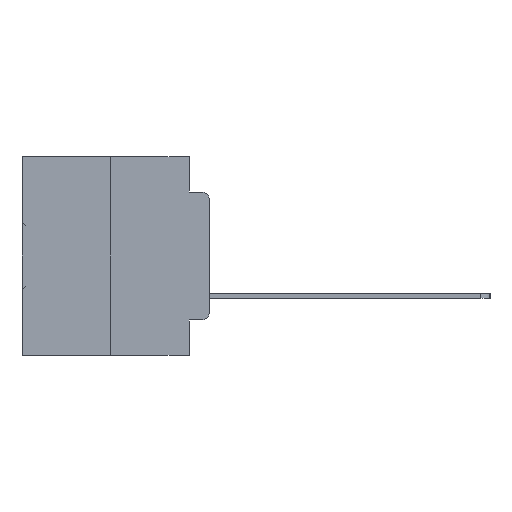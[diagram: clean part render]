
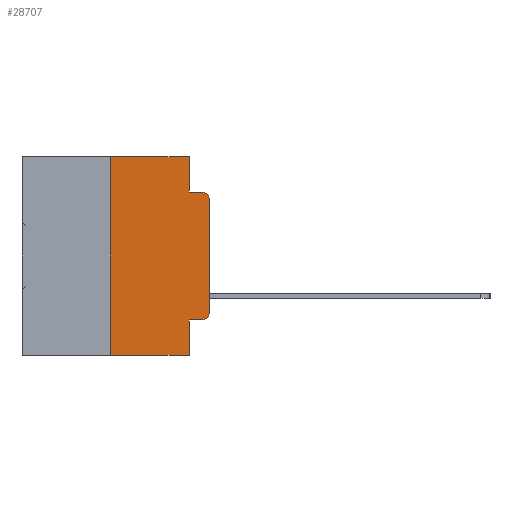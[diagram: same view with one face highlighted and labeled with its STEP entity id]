
A CAD part, left-side view. The second image highlights one B-rep face of the part: STEP entity #28707.
In plain terms, the highlighted planar face has unit normal (-1, 0, 0).
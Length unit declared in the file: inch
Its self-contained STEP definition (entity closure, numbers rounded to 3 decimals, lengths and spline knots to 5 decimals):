
#193 = CARTESIAN_POINT ( 'NONE',  ( 0., 0.051, 0. ) ) ;
#1169 = CIRCLE ( 'NONE', #34010, 0.02 ) ;
#1269 = CARTESIAN_POINT ( 'NONE',  ( 0., 0.473, 0. ) ) ;
#1538 = VECTOR ( 'NONE', #10232, 39.37008 ) ;
#2006 = AXIS2_PLACEMENT_3D ( 'NONE', #13769, #24222, #19014 ) ;
#2078 = CARTESIAN_POINT ( 'NONE',  ( 0., 0.051, -0.0885 ) ) ;
#2983 = DIRECTION ( 'NONE',  ( 0., 0., -1. ) ) ;
#3175 = VECTOR ( 'NONE', #16511, 39.37008 ) ;
#3433 = VECTOR ( 'NONE', #2983, 39.37008 ) ;
#3879 = EDGE_LOOP ( 'NONE', ( #21950, #27041, #23851, #23811, #24262, #24699, #24588, #25602, #26365, #12813 ) ) ;
#4594 = CARTESIAN_POINT ( 'NONE',  ( 0., 0.051, -0.4115 ) ) ;
#4612 = EDGE_CURVE ( 'NONE', #17593, #7597, #31254, .T. ) ;
#4682 = LINE ( 'NONE', #1269, #16323 ) ;
#6451 = EDGE_CURVE ( 'NONE', #7597, #16814, #22571, .T. ) ;
#7597 = VERTEX_POINT ( 'NONE', #2078 ) ;
#8243 = EDGE_CURVE ( 'NONE', #8988, #16814, #1169, .T. ) ;
#8244 = CARTESIAN_POINT ( 'NONE',  ( 0., 0.02, -0.1085 ) ) ;
#8622 = CARTESIAN_POINT ( 'NONE',  ( 0., 0., -0.3915 ) ) ;
#8988 = VERTEX_POINT ( 'NONE', #13660 ) ;
#9167 = CARTESIAN_POINT ( 'NONE',  ( 0., 0.02, -0.3915 ) ) ;
#10001 = LINE ( 'NONE', #22939, #23158 ) ;
#10232 = DIRECTION ( 'NONE',  ( 0., 0., 1. ) ) ;
#10560 = VERTEX_POINT ( 'NONE', #4594 ) ;
#10919 = DIRECTION ( 'NONE',  ( 0., 0., -1. ) ) ;
#11129 = CARTESIAN_POINT ( 'NONE',  ( 0., 0.25, 0. ) ) ;
#11815 = DIRECTION ( 'NONE',  ( 0., 0., -1. ) ) ;
#12265 = LINE ( 'NONE', #193, #3433 ) ;
#12270 = EDGE_CURVE ( 'NONE', #27162, #27237, #26107, .T. ) ;
#12813 = ORIENTED_EDGE ( 'NONE', *, *, #23027, .T. ) ;
#13588 = EDGE_CURVE ( 'NONE', #33265, #8988, #10001, .T. ) ;
#13660 = CARTESIAN_POINT ( 'NONE',  ( 0., 0., -0.1085 ) ) ;
#13769 = CARTESIAN_POINT ( 'NONE',  ( 0., 0.473, 0. ) ) ;
#14404 = CARTESIAN_POINT ( 'NONE',  ( 0., 0.473, -0.5 ) ) ;
#16323 = VECTOR ( 'NONE', #30356, 39.37008 ) ;
#16364 = PLANE ( 'NONE',  #2006 ) ;
#16511 = DIRECTION ( 'NONE',  ( 0., 0., -1. ) ) ;
#16645 = LINE ( 'NONE', #18410, #21992 ) ;
#16814 = VERTEX_POINT ( 'NONE', #18770 ) ;
#17593 = VERTEX_POINT ( 'NONE', #19893 ) ;
#17969 = CARTESIAN_POINT ( 'NONE',  ( 0., 0.051, -0.5 ) ) ;
#18410 = CARTESIAN_POINT ( 'NONE',  ( 0., 0.051, -0.4115 ) ) ;
#18770 = CARTESIAN_POINT ( 'NONE',  ( 0., 0.02, -0.0885 ) ) ;
#19014 = DIRECTION ( 'NONE',  ( 0., 0., -1. ) ) ;
#19676 = DIRECTION ( 'NONE',  ( 0., -1., 0. ) ) ;
#19893 = CARTESIAN_POINT ( 'NONE',  ( 0., 0.051, 0. ) ) ;
#20711 = CARTESIAN_POINT ( 'NONE',  ( 0., 0.25, 0. ) ) ;
#21300 = AXIS2_PLACEMENT_3D ( 'NONE', #9167, #27555, #11815 ) ;
#21750 = VECTOR ( 'NONE', #26437, 39.37008 ) ;
#21950 = ORIENTED_EDGE ( 'NONE', *, *, #13588, .T. ) ;
#21992 = VECTOR ( 'NONE', #23699, 39.37008 ) ;
#22571 = LINE ( 'NONE', #31605, #21750 ) ;
#22747 = VERTEX_POINT ( 'NONE', #26446 ) ;
#22797 = LINE ( 'NONE', #20711, #1538 ) ;
#22939 = CARTESIAN_POINT ( 'NONE',  ( 0., 0., 0. ) ) ;
#23027 = EDGE_CURVE ( 'NONE', #22747, #33265, #29063, .T. ) ;
#23158 = VECTOR ( 'NONE', #25599, 39.37008 ) ;
#23699 = DIRECTION ( 'NONE',  ( 0., -1., 0. ) ) ;
#23811 = ORIENTED_EDGE ( 'NONE', *, *, #4612, .F. ) ;
#23851 = ORIENTED_EDGE ( 'NONE', *, *, #6451, .F. ) ;
#24222 = DIRECTION ( 'NONE',  ( 1., 0., 0. ) ) ;
#24262 = ORIENTED_EDGE ( 'NONE', *, *, #30261, .F. ) ;
#24588 = ORIENTED_EDGE ( 'NONE', *, *, #12270, .T. ) ;
#24699 = ORIENTED_EDGE ( 'NONE', *, *, #31735, .F. ) ;
#24824 = EDGE_CURVE ( 'NONE', #10560, #22747, #16645, .T. ) ;
#25558 = CARTESIAN_POINT ( 'NONE',  ( 0., 0.25, -0.5 ) ) ;
#25599 = DIRECTION ( 'NONE',  ( 0., 0., 1. ) ) ;
#25602 = ORIENTED_EDGE ( 'NONE', *, *, #30017, .F. ) ;
#26107 = LINE ( 'NONE', #14404, #32154 ) ;
#26365 = ORIENTED_EDGE ( 'NONE', *, *, #24824, .T. ) ;
#26437 = DIRECTION ( 'NONE',  ( 0., -1., 0. ) ) ;
#26446 = CARTESIAN_POINT ( 'NONE',  ( 0., 0.02, -0.4115 ) ) ;
#26676 = DIRECTION ( 'NONE',  ( -1., 0., 0. ) ) ;
#27041 = ORIENTED_EDGE ( 'NONE', *, *, #8243, .T. ) ;
#27162 = VERTEX_POINT ( 'NONE', #25558 ) ;
#27237 = VERTEX_POINT ( 'NONE', #17969 ) ;
#27555 = DIRECTION ( 'NONE',  ( -1., 0., 0. ) ) ;
#28629 = FACE_OUTER_BOUND ( 'NONE', #3879, .T. ) ;
#28707 = ADVANCED_FACE ( 'NONE', ( #28629 ), #16364, .F. ) ;
#29063 = CIRCLE ( 'NONE', #21300, 0.02 ) ;
#29576 = CARTESIAN_POINT ( 'NONE',  ( 0., 0.051, 0. ) ) ;
#30017 = EDGE_CURVE ( 'NONE', #10560, #27237, #12265, .T. ) ;
#30029 = VERTEX_POINT ( 'NONE', #11129 ) ;
#30261 = EDGE_CURVE ( 'NONE', #30029, #17593, #4682, .T. ) ;
#30356 = DIRECTION ( 'NONE',  ( 0., -1., 0. ) ) ;
#31254 = LINE ( 'NONE', #29576, #3175 ) ;
#31605 = CARTESIAN_POINT ( 'NONE',  ( 0., 0.051, -0.0885 ) ) ;
#31735 = EDGE_CURVE ( 'NONE', #27162, #30029, #22797, .T. ) ;
#32154 = VECTOR ( 'NONE', #19676, 39.37008 ) ;
#33265 = VERTEX_POINT ( 'NONE', #8622 ) ;
#34010 = AXIS2_PLACEMENT_3D ( 'NONE', #8244, #26676, #10919 ) ;
